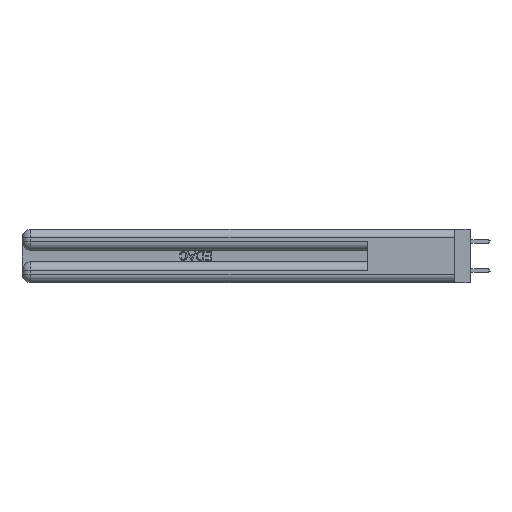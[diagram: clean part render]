
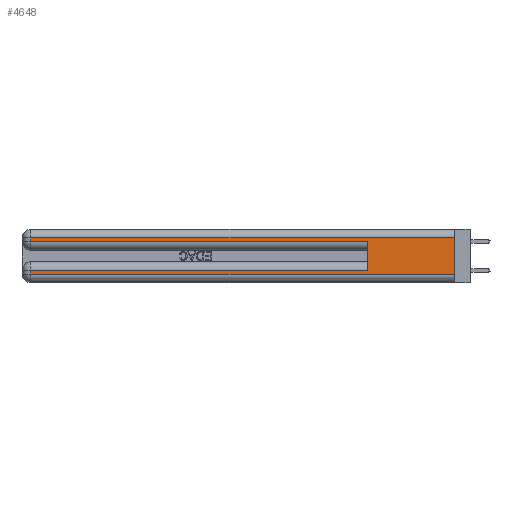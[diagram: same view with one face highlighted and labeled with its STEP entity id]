
A CAD part, left-side view. The second image highlights one B-rep face of the part: STEP entity #4648.
In plain terms, the highlighted planar face has unit normal (-1, 0, 0).
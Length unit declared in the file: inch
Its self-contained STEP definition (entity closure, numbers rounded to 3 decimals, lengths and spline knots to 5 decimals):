
#1184 = EDGE_CURVE ( 'NONE', #4756, #32574, #17880, .T. ) ;
#1548 = ORIENTED_EDGE ( 'NONE', *, *, #15987, .T. ) ;
#2643 = LINE ( 'NONE', #32872, #7123 ) ;
#3639 = DIRECTION ( 'NONE',  ( 0., 0., -1. ) ) ;
#3931 = CARTESIAN_POINT ( 'NONE',  ( 0., 0., 0.31 ) ) ;
#4648 = ADVANCED_FACE ( 'NONE', ( #42081 ), #32406, .F. ) ;
#4756 = VERTEX_POINT ( 'NONE', #9450 ) ;
#4937 = DIRECTION ( 'NONE',  ( 0., 0., -1. ) ) ;
#5260 = CARTESIAN_POINT ( 'NONE',  ( 0., 2.94, 0.37 ) ) ;
#7123 = VECTOR ( 'NONE', #43974, 39.37008 ) ;
#8005 = CARTESIAN_POINT ( 'NONE',  ( 0., 0., 0.31 ) ) ;
#8173 = VERTEX_POINT ( 'NONE', #37124 ) ;
#8434 = ORIENTED_EDGE ( 'NONE', *, *, #28372, .T. ) ;
#9450 = CARTESIAN_POINT ( 'NONE',  ( 0., 2.94, 0.06 ) ) ;
#9480 = DIRECTION ( 'NONE',  ( 0., 1., 0. ) ) ;
#12174 = VECTOR ( 'NONE', #36271, 39.37008 ) ;
#12295 = VERTEX_POINT ( 'NONE', #14019 ) ;
#13416 = CARTESIAN_POINT ( 'NONE',  ( 0., 2.94, 0.085 ) ) ;
#14019 = CARTESIAN_POINT ( 'NONE',  ( 0., 2.94, 0.31 ) ) ;
#14542 = CARTESIAN_POINT ( 'NONE',  ( 0., 0.6, 0.285 ) ) ;
#14905 = AXIS2_PLACEMENT_3D ( 'NONE', #40009, #18947, #29449 ) ;
#15966 = VECTOR ( 'NONE', #3639, 39.37008 ) ;
#15987 = EDGE_CURVE ( 'NONE', #18242, #4756, #2643, .T. ) ;
#17588 = ORIENTED_EDGE ( 'NONE', *, *, #30815, .F. ) ;
#17880 = LINE ( 'NONE', #37301, #44563 ) ;
#18091 = CARTESIAN_POINT ( 'NONE',  ( 0., 0.6, 0.085 ) ) ;
#18242 = VERTEX_POINT ( 'NONE', #13416 ) ;
#18564 = EDGE_LOOP ( 'NONE', ( #17588, #27671, #30502, #26167, #19241, #8434, #1548, #20831 ) ) ;
#18576 = EDGE_CURVE ( 'NONE', #8173, #31277, #30826, .T. ) ;
#18586 = CARTESIAN_POINT ( 'NONE',  ( 0., 0.6, 0.145 ) ) ;
#18947 = DIRECTION ( 'NONE',  ( 1., 0., 0. ) ) ;
#19241 = ORIENTED_EDGE ( 'NONE', *, *, #23162, .F. ) ;
#19260 = LINE ( 'NONE', #5260, #45392 ) ;
#20831 = ORIENTED_EDGE ( 'NONE', *, *, #1184, .T. ) ;
#21905 = EDGE_CURVE ( 'NONE', #12295, #8173, #19260, .T. ) ;
#23153 = LINE ( 'NONE', #28673, #15966 ) ;
#23162 = EDGE_CURVE ( 'NONE', #40886, #31277, #24786, .T. ) ;
#24786 = LINE ( 'NONE', #18586, #31421 ) ;
#24801 = DIRECTION ( 'NONE',  ( 0., 0., 1. ) ) ;
#26167 = ORIENTED_EDGE ( 'NONE', *, *, #18576, .T. ) ;
#27671 = ORIENTED_EDGE ( 'NONE', *, *, #28799, .T. ) ;
#28270 = DIRECTION ( 'NONE',  ( 0., -1., 0. ) ) ;
#28372 = EDGE_CURVE ( 'NONE', #40886, #18242, #30528, .T. ) ;
#28673 = CARTESIAN_POINT ( 'NONE',  ( 0., 0., 0.37 ) ) ;
#28799 = EDGE_CURVE ( 'NONE', #30734, #12295, #30482, .T. ) ;
#29449 = DIRECTION ( 'NONE',  ( 0., 0., -1. ) ) ;
#30482 = LINE ( 'NONE', #8005, #12174 ) ;
#30502 = ORIENTED_EDGE ( 'NONE', *, *, #21905, .T. ) ;
#30528 = LINE ( 'NONE', #30772, #33845 ) ;
#30734 = VERTEX_POINT ( 'NONE', #3931 ) ;
#30736 = CARTESIAN_POINT ( 'NONE',  ( 0., 0., 0.06 ) ) ;
#30772 = CARTESIAN_POINT ( 'NONE',  ( 0., 0., 0.085 ) ) ;
#30815 = EDGE_CURVE ( 'NONE', #30734, #32574, #23153, .T. ) ;
#30826 = LINE ( 'NONE', #35248, #40831 ) ;
#31277 = VERTEX_POINT ( 'NONE', #14542 ) ;
#31421 = VECTOR ( 'NONE', #24801, 39.37008 ) ;
#32406 = PLANE ( 'NONE',  #14905 ) ;
#32574 = VERTEX_POINT ( 'NONE', #30736 ) ;
#32872 = CARTESIAN_POINT ( 'NONE',  ( 0., 2.94, 0.37 ) ) ;
#33845 = VECTOR ( 'NONE', #9480, 39.37008 ) ;
#35248 = CARTESIAN_POINT ( 'NONE',  ( 0., 0., 0.285 ) ) ;
#35674 = DIRECTION ( 'NONE',  ( 0., -1., 0. ) ) ;
#36271 = DIRECTION ( 'NONE',  ( 0., 1., 0. ) ) ;
#37124 = CARTESIAN_POINT ( 'NONE',  ( 0., 2.94, 0.285 ) ) ;
#37301 = CARTESIAN_POINT ( 'NONE',  ( 0., 0., 0.06 ) ) ;
#40009 = CARTESIAN_POINT ( 'NONE',  ( 0., 0., 0.37 ) ) ;
#40831 = VECTOR ( 'NONE', #28270, 39.37008 ) ;
#40886 = VERTEX_POINT ( 'NONE', #18091 ) ;
#42081 = FACE_OUTER_BOUND ( 'NONE', #18564, .T. ) ;
#43974 = DIRECTION ( 'NONE',  ( 0., 0., -1. ) ) ;
#44563 = VECTOR ( 'NONE', #35674, 39.37008 ) ;
#45392 = VECTOR ( 'NONE', #4937, 39.37008 ) ;
